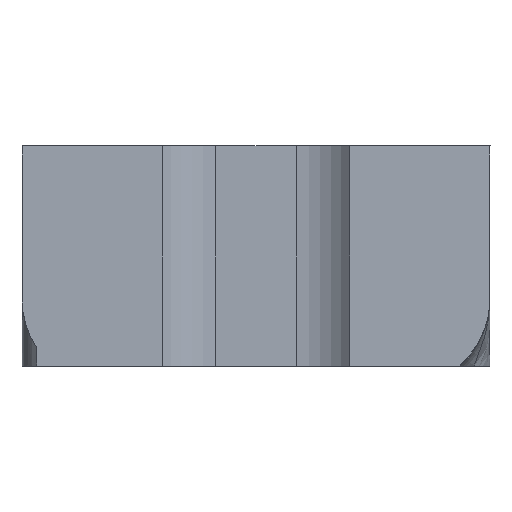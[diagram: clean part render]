
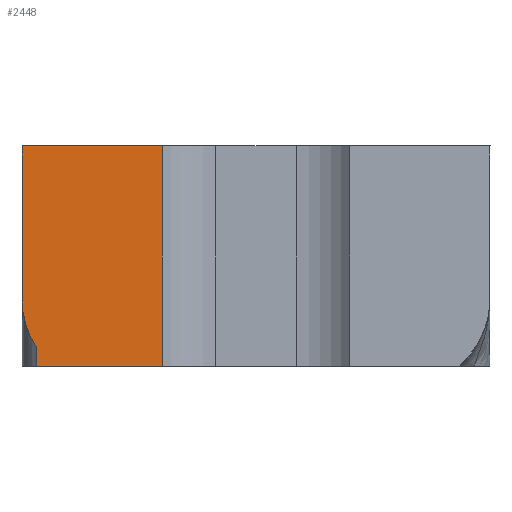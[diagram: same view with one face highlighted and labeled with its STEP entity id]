
A CAD part, left-side view. The second image highlights one B-rep face of the part: STEP entity #2448.
In plain terms, the highlighted planar face has unit normal (-1, 0, 0).
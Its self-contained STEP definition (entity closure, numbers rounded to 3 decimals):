
#172 = LINE ( 'NONE', #942, #1027 ) ;
#175 = CARTESIAN_POINT ( 'NONE',  ( 82.199, -4.883, -3.647 ) ) ;
#182 = ORIENTED_EDGE ( 'NONE', *, *, #2518, .T. ) ;
#269 = CARTESIAN_POINT ( 'NONE',  ( 82.199, 5.066, 7.452 ) ) ;
#422 = EDGE_CURVE ( 'NONE', #2590, #1177, #769, .T. ) ;
#479 = DIRECTION ( 'NONE',  ( 1., 0., 0. ) ) ;
#508 = DIRECTION ( 'NONE',  ( 0., 0., 1. ) ) ;
#522 = ORIENTED_EDGE ( 'NONE', *, *, #826, .T. ) ;
#550 = VECTOR ( 'NONE', #2758, 1000. ) ;
#657 = ORIENTED_EDGE ( 'NONE', *, *, #1824, .T. ) ;
#695 = DIRECTION ( 'NONE',  ( 0., 0., -1. ) ) ;
#769 = LINE ( 'NONE', #2917, #1381 ) ;
#789 = LINE ( 'NONE', #2935, #2660 ) ;
#826 = EDGE_CURVE ( 'NONE', #1531, #1177, #893, .T. ) ;
#868 = ORIENTED_EDGE ( 'NONE', *, *, #1951, .F. ) ;
#872 = VERTEX_POINT ( 'NONE', #1479 ) ;
#893 = LINE ( 'NONE', #3352, #550 ) ;
#942 = CARTESIAN_POINT ( 'NONE',  ( 82.199, -4.883, -17.935 ) ) ;
#1000 = LINE ( 'NONE', #269, #3328 ) ;
#1018 = DIRECTION ( 'NONE',  ( 0., 0., -1. ) ) ;
#1023 = AXIS2_PLACEMENT_3D ( 'NONE', #1916, #1633, #1652 ) ;
#1027 = VECTOR ( 'NONE', #695, 1000. ) ;
#1177 = VERTEX_POINT ( 'NONE', #2196 ) ;
#1354 = EDGE_LOOP ( 'NONE', ( #522, #2978, #182, #2522, #657, #868 ) ) ;
#1381 = VECTOR ( 'NONE', #508, 1000. ) ;
#1392 = CARTESIAN_POINT ( 'NONE',  ( 82.199, 5.066, -2.19 ) ) ;
#1479 = CARTESIAN_POINT ( 'NONE',  ( 82.199, 5.066, -3.647 ) ) ;
#1531 = VERTEX_POINT ( 'NONE', #1584 ) ;
#1534 = FACE_OUTER_BOUND ( 'NONE', #1354, .T. ) ;
#1550 = DIRECTION ( 'NONE',  ( 0., 1., 0. ) ) ;
#1584 = CARTESIAN_POINT ( 'NONE',  ( 82.199, -4.883, 13.815 ) ) ;
#1633 = DIRECTION ( 'NONE',  ( -1., 0., 0. ) ) ;
#1652 = DIRECTION ( 'NONE',  ( 0., 1., 0. ) ) ;
#1732 = CARTESIAN_POINT ( 'NONE',  ( 82.199, 6.232, 1.695 ) ) ;
#1814 = CARTESIAN_POINT ( 'NONE',  ( 82.199, 69.175, 17.442 ) ) ;
#1824 = EDGE_CURVE ( 'NONE', #872, #2644, #789, .T. ) ;
#1864 = DIRECTION ( 'NONE',  ( 0., -1., 0. ) ) ;
#1916 = CARTESIAN_POINT ( 'NONE',  ( 82.199, -0.825, 1.695 ) ) ;
#1951 = EDGE_CURVE ( 'NONE', #1531, #2644, #172, .T. ) ;
#2073 = VERTEX_POINT ( 'NONE', #1392 ) ;
#2083 = PLANE ( 'NONE',  #3168 ) ;
#2196 = CARTESIAN_POINT ( 'NONE',  ( 82.199, 6.232, 13.815 ) ) ;
#2448 = ADVANCED_FACE ( 'NONE', ( #1534 ), #2083, .F. ) ;
#2518 = EDGE_CURVE ( 'NONE', #2590, #2073, #3159, .T. ) ;
#2522 = ORIENTED_EDGE ( 'NONE', *, *, #2734, .T. ) ;
#2590 = VERTEX_POINT ( 'NONE', #1732 ) ;
#2644 = VERTEX_POINT ( 'NONE', #175 ) ;
#2660 = VECTOR ( 'NONE', #1864, 1000. ) ;
#2734 = EDGE_CURVE ( 'NONE', #2073, #872, #1000, .T. ) ;
#2758 = DIRECTION ( 'NONE',  ( 0., 1., 0. ) ) ;
#2917 = CARTESIAN_POINT ( 'NONE',  ( 82.199, 6.232, 1.695 ) ) ;
#2935 = CARTESIAN_POINT ( 'NONE',  ( 82.199, 69.175, -3.647 ) ) ;
#2978 = ORIENTED_EDGE ( 'NONE', *, *, #422, .F. ) ;
#3159 = CIRCLE ( 'NONE', #1023, 7.057 ) ;
#3168 = AXIS2_PLACEMENT_3D ( 'NONE', #1814, #479, #1550 ) ;
#3328 = VECTOR ( 'NONE', #1018, 1000. ) ;
#3352 = CARTESIAN_POINT ( 'NONE',  ( 82.199, 69.175, 13.815 ) ) ;
